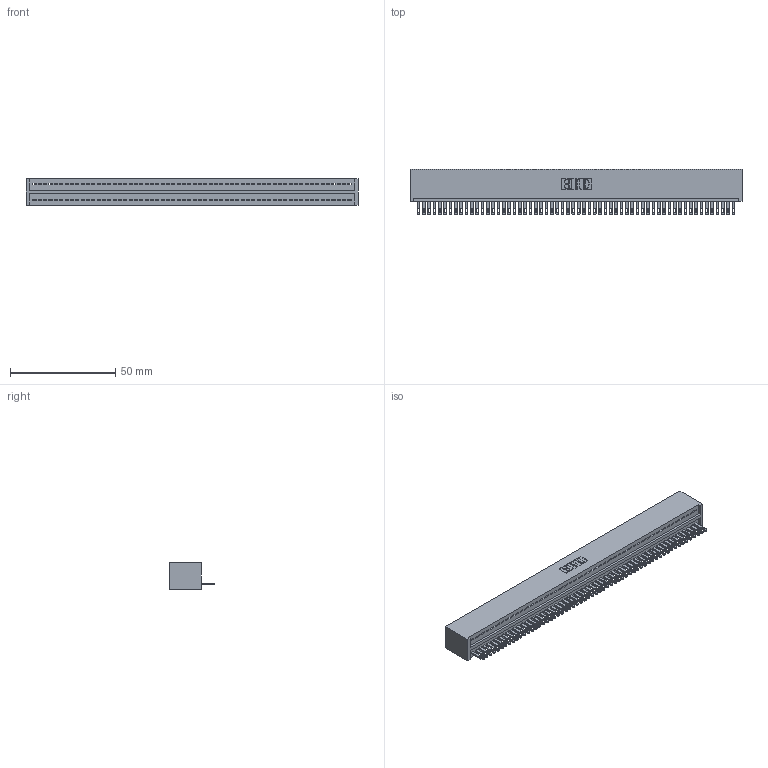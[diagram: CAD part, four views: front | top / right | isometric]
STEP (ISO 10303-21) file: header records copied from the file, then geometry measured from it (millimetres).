
FILE_DESCRIPTION (( 'STEP AP203' ), '1' );
FILE_NAME ('325-060-500-101.STEP', '2020-02-25T02:21:15', ( '' ), ( '' ), 'SwSTEP 2.0', 'SolidWorks 2016', '' );
FILE_SCHEMA (( 'CONFIG_CONTROL_DESIGN' ));
Length unit declared in the file: inch
Products named in the file (3): 325 Part_Lugless; 325-292-001_325-293-100; 325-060-500-101
Assembly tree (61 placements, depth 2):
  325-060-500-101
    325 Part_Lugless
    325-292-001_325-293-100  x60
Bounding box: 158.04 x 21.84 x 12.45 mm (x, y, z)
Volume: 20813.5 mm3; surface area: 23674.9 mm2
Topology: 61 solids, 61 shells, 3346 faces, 10367 edges, 6910 vertices
Faces by surface type: plane 2226, cylinder 1120
Entity records: 34005 total; most frequent: CARTESIAN_POINT 5870, ORIENTED_EDGE 5866, DIRECTION 4909, EDGE_CURVE 2933, LINE 2809, VECTOR 2809, VERTEX_POINT 1954, AXIS2_PLACEMENT_3D 1050
